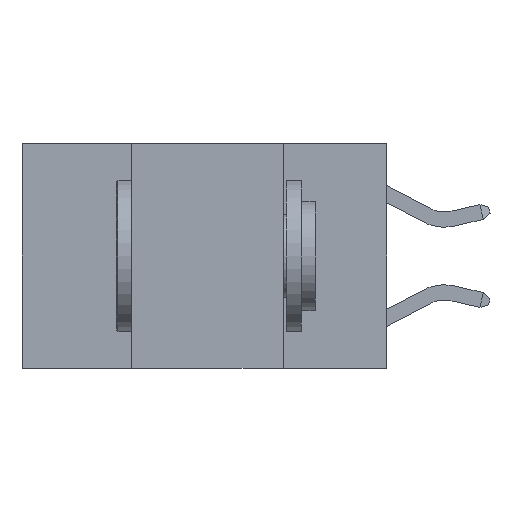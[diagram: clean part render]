
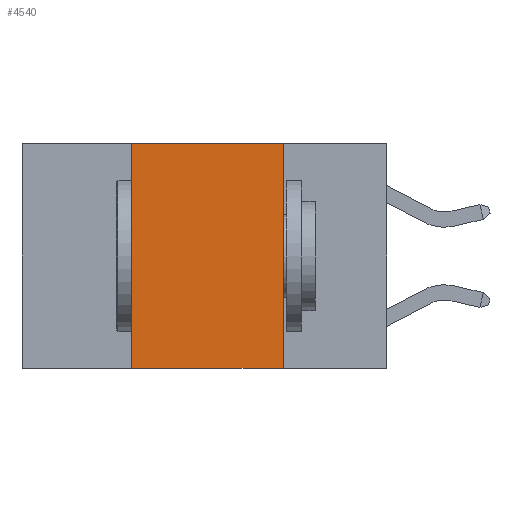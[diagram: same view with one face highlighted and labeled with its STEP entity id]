
A CAD part, left-side view. The second image highlights one B-rep face of the part: STEP entity #4540.
In plain terms, the highlighted planar face has unit normal (-1, 0, 0).
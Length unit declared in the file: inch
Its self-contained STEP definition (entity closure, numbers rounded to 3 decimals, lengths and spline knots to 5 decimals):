
#107 = CARTESIAN_POINT ( 'NONE',  ( 0., 0.17, 0. ) ) ;
#485 = VECTOR ( 'NONE', #9944, 39.37008 ) ;
#857 = VECTOR ( 'NONE', #9656, 39.37008 ) ;
#879 = EDGE_CURVE ( 'NONE', #12175, #15491, #12962, .T. ) ;
#1035 = DIRECTION ( 'NONE',  ( 0., 0., -1. ) ) ;
#1291 = LINE ( 'NONE', #15991, #485 ) ;
#1435 = CARTESIAN_POINT ( 'NONE',  ( 0., 0.6, 0. ) ) ;
#1935 = EDGE_CURVE ( 'NONE', #14691, #11282, #3922, .T. ) ;
#2191 = FACE_OUTER_BOUND ( 'NONE', #12993, .T. ) ;
#2213 = CARTESIAN_POINT ( 'NONE',  ( 0., 0.42, 0. ) ) ;
#2443 = EDGE_CURVE ( 'NONE', #11282, #12175, #5247, .T. ) ;
#3135 = VECTOR ( 'NONE', #1035, 39.37008 ) ;
#3345 = CARTESIAN_POINT ( 'NONE',  ( 0., 0.42, 0. ) ) ;
#3922 = LINE ( 'NONE', #2213, #857 ) ;
#4059 = DIRECTION ( 'NONE',  ( 1., 0., 0. ) ) ;
#4540 = ADVANCED_FACE ( 'NONE', ( #2191 ), #7754, .F. ) ;
#4869 = VECTOR ( 'NONE', #4898, 39.37008 ) ;
#4898 = DIRECTION ( 'NONE',  ( 0., -1., 0. ) ) ;
#5247 = LINE ( 'NONE', #8569, #4869 ) ;
#5842 = CARTESIAN_POINT ( 'NONE',  ( 0., 0.17, -0.37 ) ) ;
#5856 = ORIENTED_EDGE ( 'NONE', *, *, #879, .F. ) ;
#7754 = PLANE ( 'NONE',  #14043 ) ;
#8120 = CARTESIAN_POINT ( 'NONE',  ( 0., 0.17, 0. ) ) ;
#8569 = CARTESIAN_POINT ( 'NONE',  ( 0., 0.6, 0. ) ) ;
#9656 = DIRECTION ( 'NONE',  ( 0., 0., 1. ) ) ;
#9944 = DIRECTION ( 'NONE',  ( 0., -1., 0. ) ) ;
#11282 = VERTEX_POINT ( 'NONE', #3345 ) ;
#11737 = ORIENTED_EDGE ( 'NONE', *, *, #2443, .F. ) ;
#12175 = VERTEX_POINT ( 'NONE', #107 ) ;
#12626 = DIRECTION ( 'NONE',  ( 0., 0., -1. ) ) ;
#12690 = ORIENTED_EDGE ( 'NONE', *, *, #1935, .F. ) ;
#12707 = ORIENTED_EDGE ( 'NONE', *, *, #15132, .T. ) ;
#12962 = LINE ( 'NONE', #8120, #3135 ) ;
#12993 = EDGE_LOOP ( 'NONE', ( #5856, #11737, #12690, #12707 ) ) ;
#14043 = AXIS2_PLACEMENT_3D ( 'NONE', #1435, #4059, #12626 ) ;
#14691 = VERTEX_POINT ( 'NONE', #15380 ) ;
#15132 = EDGE_CURVE ( 'NONE', #14691, #15491, #1291, .T. ) ;
#15380 = CARTESIAN_POINT ( 'NONE',  ( 0., 0.42, -0.37 ) ) ;
#15491 = VERTEX_POINT ( 'NONE', #5842 ) ;
#15991 = CARTESIAN_POINT ( 'NONE',  ( 0., 0.6, -0.37 ) ) ;
